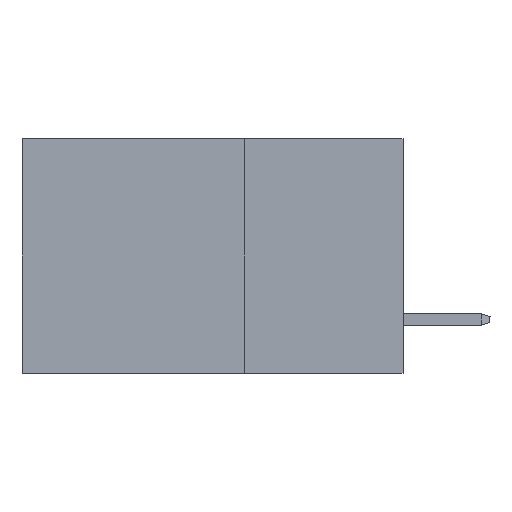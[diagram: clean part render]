
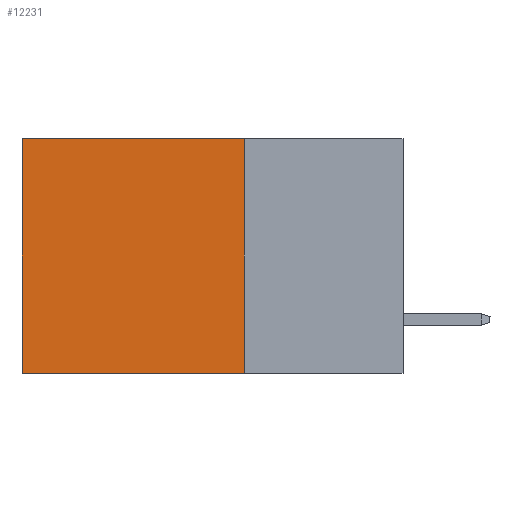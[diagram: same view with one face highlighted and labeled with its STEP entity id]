
A CAD part, left-side view. The second image highlights one B-rep face of the part: STEP entity #12231.
In plain terms, the highlighted planar face has unit normal (-1, 0, 0).
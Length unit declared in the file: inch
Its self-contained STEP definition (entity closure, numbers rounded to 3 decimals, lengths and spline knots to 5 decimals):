
#726 = VERTEX_POINT ( 'NONE', #7274 ) ;
#1252 = ORIENTED_EDGE ( 'NONE', *, *, #1910, .F. ) ;
#1910 = EDGE_CURVE ( 'NONE', #10891, #726, #12769, .T. ) ;
#2690 = CARTESIAN_POINT ( 'NONE',  ( 0.2875, 0.25, -0.37 ) ) ;
#3111 = CARTESIAN_POINT ( 'NONE',  ( 0.2875, 0.25, -0.37 ) ) ;
#3746 = DIRECTION ( 'NONE',  ( 0., 0., -1. ) ) ;
#4275 = CARTESIAN_POINT ( 'NONE',  ( 0.2875, 0.25, 0. ) ) ;
#4314 = CARTESIAN_POINT ( 'NONE',  ( 0.2875, 0.25, 0. ) ) ;
#5413 = CARTESIAN_POINT ( 'NONE',  ( 0.2875, 0.6, 0. ) ) ;
#6723 = EDGE_CURVE ( 'NONE', #11154, #10891, #9413, .T. ) ;
#7064 = CARTESIAN_POINT ( 'NONE',  ( 0.2875, 0.25, 0. ) ) ;
#7260 = ORIENTED_EDGE ( 'NONE', *, *, #21156, .T. ) ;
#7274 = CARTESIAN_POINT ( 'NONE',  ( 0.2875, 0.6, -0.37 ) ) ;
#7713 = VECTOR ( 'NONE', #17467, 39.37008 ) ;
#8253 = DIRECTION ( 'NONE',  ( 1., 0., 0. ) ) ;
#8941 = VERTEX_POINT ( 'NONE', #14319 ) ;
#9289 = VECTOR ( 'NONE', #9344, 39.37008 ) ;
#9344 = DIRECTION ( 'NONE',  ( 0., 1., 0. ) ) ;
#9413 = LINE ( 'NONE', #4275, #10528 ) ;
#10101 = ORIENTED_EDGE ( 'NONE', *, *, #18849, .T. ) ;
#10268 = ORIENTED_EDGE ( 'NONE', *, *, #6723, .F. ) ;
#10528 = VECTOR ( 'NONE', #15951, 39.37008 ) ;
#10891 = VERTEX_POINT ( 'NONE', #2690 ) ;
#11154 = VERTEX_POINT ( 'NONE', #7064 ) ;
#11693 = CARTESIAN_POINT ( 'NONE',  ( 0.2875, 0.25, 0. ) ) ;
#11888 = AXIS2_PLACEMENT_3D ( 'NONE', #11693, #8253, #3746 ) ;
#11904 = FACE_OUTER_BOUND ( 'NONE', #19722, .T. ) ;
#12231 = ADVANCED_FACE ( 'NONE', ( #11904 ), #18427, .F. ) ;
#12302 = DIRECTION ( 'NONE',  ( 0., 0., -1. ) ) ;
#12769 = LINE ( 'NONE', #3111, #7713 ) ;
#14319 = CARTESIAN_POINT ( 'NONE',  ( 0.2875, 0.6, 0. ) ) ;
#14594 = LINE ( 'NONE', #4314, #9289 ) ;
#15951 = DIRECTION ( 'NONE',  ( 0., 0., -1. ) ) ;
#17097 = LINE ( 'NONE', #5413, #20666 ) ;
#17467 = DIRECTION ( 'NONE',  ( 0., 1., 0. ) ) ;
#18427 = PLANE ( 'NONE',  #11888 ) ;
#18849 = EDGE_CURVE ( 'NONE', #11154, #8941, #14594, .T. ) ;
#19722 = EDGE_LOOP ( 'NONE', ( #7260, #1252, #10268, #10101 ) ) ;
#20666 = VECTOR ( 'NONE', #12302, 39.37008 ) ;
#21156 = EDGE_CURVE ( 'NONE', #8941, #726, #17097, .T. ) ;
